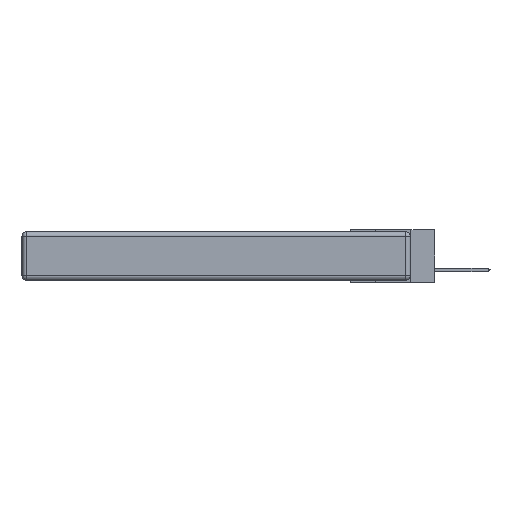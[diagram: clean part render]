
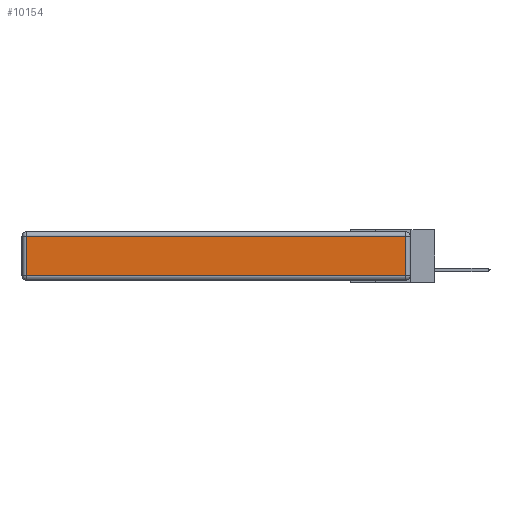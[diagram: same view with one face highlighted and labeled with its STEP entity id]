
A CAD part, left-side view. The second image highlights one B-rep face of the part: STEP entity #10154.
In plain terms, the highlighted planar face has unit normal (-1, 0, 0).
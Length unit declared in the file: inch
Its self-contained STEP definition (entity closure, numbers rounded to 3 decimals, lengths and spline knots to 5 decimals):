
#31 = DIRECTION ( 'NONE',  ( 0., 0., 1. ) ) ;
#203 = CARTESIAN_POINT ( 'NONE',  ( 0., 0.03, -0.343 ) ) ;
#414 = LINE ( 'NONE', #9170, #7641 ) ;
#453 = DIRECTION ( 'NONE',  ( 0., 0., -1. ) ) ;
#582 = CARTESIAN_POINT ( 'NONE',  ( 0., 0.03, -0.03 ) ) ;
#1656 = EDGE_CURVE ( 'NONE', #14494, #13420, #10157, .T. ) ;
#2483 = EDGE_LOOP ( 'NONE', ( #11931, #17546, #6513, #16008 ) ) ;
#3448 = EDGE_CURVE ( 'NONE', #13911, #9078, #8871, .T. ) ;
#5000 = DIRECTION ( 'NONE',  ( -1., 0., 0. ) ) ;
#5376 = FACE_OUTER_BOUND ( 'NONE', #2483, .T. ) ;
#5673 = VECTOR ( 'NONE', #19819, 39.37008 ) ;
#6194 = LINE ( 'NONE', #203, #5673 ) ;
#6280 = DIRECTION ( 'NONE',  ( 0., 1., 0. ) ) ;
#6513 = ORIENTED_EDGE ( 'NONE', *, *, #3448, .T. ) ;
#7641 = VECTOR ( 'NONE', #453, 39.37008 ) ;
#8871 = LINE ( 'NONE', #11332, #10406 ) ;
#9078 = VERTEX_POINT ( 'NONE', #17316 ) ;
#9170 = CARTESIAN_POINT ( 'NONE',  ( 0., 2.72, -0.343 ) ) ;
#9623 = CARTESIAN_POINT ( 'NONE',  ( 0., 2.72, -0.313 ) ) ;
#9777 = EDGE_CURVE ( 'NONE', #13420, #13911, #6194, .T. ) ;
#10154 = ADVANCED_FACE ( 'NONE', ( #5376 ), #14796, .T. ) ;
#10157 = LINE ( 'NONE', #18013, #14008 ) ;
#10406 = VECTOR ( 'NONE', #6280, 39.37008 ) ;
#11332 = CARTESIAN_POINT ( 'NONE',  ( 0., 2.75, -0.03 ) ) ;
#11573 = CARTESIAN_POINT ( 'NONE',  ( 0., 0., -0.343 ) ) ;
#11931 = ORIENTED_EDGE ( 'NONE', *, *, #1656, .T. ) ;
#13420 = VERTEX_POINT ( 'NONE', #17554 ) ;
#13911 = VERTEX_POINT ( 'NONE', #582 ) ;
#14008 = VECTOR ( 'NONE', #17246, 39.37008 ) ;
#14494 = VERTEX_POINT ( 'NONE', #9623 ) ;
#14796 = PLANE ( 'NONE',  #16542 ) ;
#16008 = ORIENTED_EDGE ( 'NONE', *, *, #17036, .T. ) ;
#16542 = AXIS2_PLACEMENT_3D ( 'NONE', #11573, #5000, #31 ) ;
#17036 = EDGE_CURVE ( 'NONE', #9078, #14494, #414, .T. ) ;
#17246 = DIRECTION ( 'NONE',  ( 0., -1., 0. ) ) ;
#17316 = CARTESIAN_POINT ( 'NONE',  ( 0., 2.72, -0.03 ) ) ;
#17546 = ORIENTED_EDGE ( 'NONE', *, *, #9777, .T. ) ;
#17554 = CARTESIAN_POINT ( 'NONE',  ( 0., 0.03, -0.313 ) ) ;
#18013 = CARTESIAN_POINT ( 'NONE',  ( 0., 0., -0.313 ) ) ;
#19819 = DIRECTION ( 'NONE',  ( 0., 0., 1. ) ) ;
